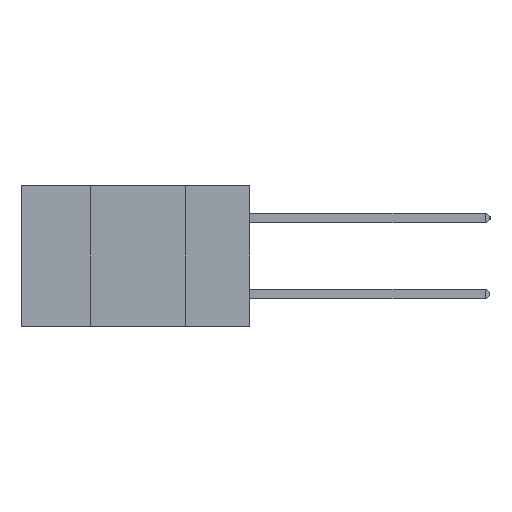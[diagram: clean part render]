
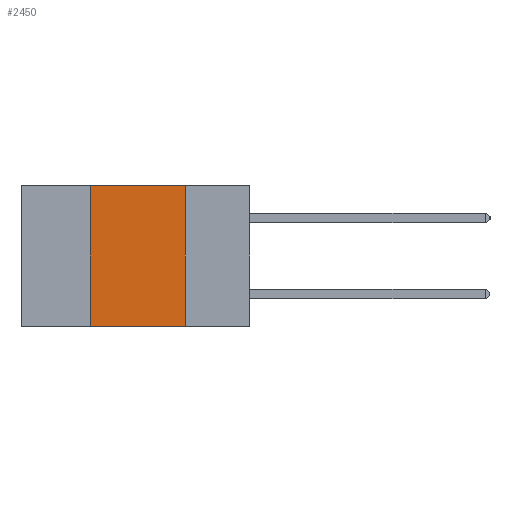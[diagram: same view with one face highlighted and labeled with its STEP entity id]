
A CAD part, left-side view. The second image highlights one B-rep face of the part: STEP entity #2450.
In plain terms, the highlighted planar face has unit normal (-1, 0, 0).
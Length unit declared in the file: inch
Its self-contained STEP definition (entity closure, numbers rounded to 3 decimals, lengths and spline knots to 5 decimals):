
#994 = CARTESIAN_POINT ( 'NONE',  ( 0., 0.17, -0.37 ) ) ;
#1614 = LINE ( 'NONE', #9460, #12849 ) ;
#1720 = LINE ( 'NONE', #7160, #5297 ) ;
#1786 = ORIENTED_EDGE ( 'NONE', *, *, #9510, .F. ) ;
#2450 = ADVANCED_FACE ( 'NONE', ( #3883 ), #5570, .F. ) ;
#2978 = VERTEX_POINT ( 'NONE', #994 ) ;
#3883 = FACE_OUTER_BOUND ( 'NONE', #3965, .T. ) ;
#3965 = EDGE_LOOP ( 'NONE', ( #4175, #15638, #1786, #4893 ) ) ;
#4175 = ORIENTED_EDGE ( 'NONE', *, *, #5397, .F. ) ;
#4620 = DIRECTION ( 'NONE',  ( 0., 0., 1. ) ) ;
#4893 = ORIENTED_EDGE ( 'NONE', *, *, #12845, .T. ) ;
#5196 = EDGE_CURVE ( 'NONE', #6387, #14826, #5539, .T. ) ;
#5297 = VECTOR ( 'NONE', #8192, 39.37008 ) ;
#5397 = EDGE_CURVE ( 'NONE', #14826, #2978, #1720, .T. ) ;
#5539 = LINE ( 'NONE', #17229, #13152 ) ;
#5570 = PLANE ( 'NONE',  #15361 ) ;
#6387 = VERTEX_POINT ( 'NONE', #17253 ) ;
#6862 = CARTESIAN_POINT ( 'NONE',  ( 0., 0.6, 0. ) ) ;
#7160 = CARTESIAN_POINT ( 'NONE',  ( 0., 0.17, 0. ) ) ;
#7244 = DIRECTION ( 'NONE',  ( 1., 0., 0. ) ) ;
#7246 = DIRECTION ( 'NONE',  ( 0., 0., -1. ) ) ;
#8192 = DIRECTION ( 'NONE',  ( 0., 0., -1. ) ) ;
#8434 = DIRECTION ( 'NONE',  ( 0., -1., 0. ) ) ;
#8880 = CARTESIAN_POINT ( 'NONE',  ( 0., 0.42, -0.37 ) ) ;
#8936 = VERTEX_POINT ( 'NONE', #8880 ) ;
#9460 = CARTESIAN_POINT ( 'NONE',  ( 0., 0.6, -0.37 ) ) ;
#9510 = EDGE_CURVE ( 'NONE', #8936, #6387, #15899, .T. ) ;
#10906 = DIRECTION ( 'NONE',  ( 0., -1., 0. ) ) ;
#12543 = VECTOR ( 'NONE', #4620, 39.37008 ) ;
#12845 = EDGE_CURVE ( 'NONE', #8936, #2978, #1614, .T. ) ;
#12849 = VECTOR ( 'NONE', #10906, 39.37008 ) ;
#13152 = VECTOR ( 'NONE', #8434, 39.37008 ) ;
#13212 = CARTESIAN_POINT ( 'NONE',  ( 0., 0.42, 0. ) ) ;
#14826 = VERTEX_POINT ( 'NONE', #18018 ) ;
#15361 = AXIS2_PLACEMENT_3D ( 'NONE', #6862, #7244, #7246 ) ;
#15638 = ORIENTED_EDGE ( 'NONE', *, *, #5196, .F. ) ;
#15899 = LINE ( 'NONE', #13212, #12543 ) ;
#17229 = CARTESIAN_POINT ( 'NONE',  ( 0., 0.6, 0. ) ) ;
#17253 = CARTESIAN_POINT ( 'NONE',  ( 0., 0.42, 0. ) ) ;
#18018 = CARTESIAN_POINT ( 'NONE',  ( 0., 0.17, 0. ) ) ;
